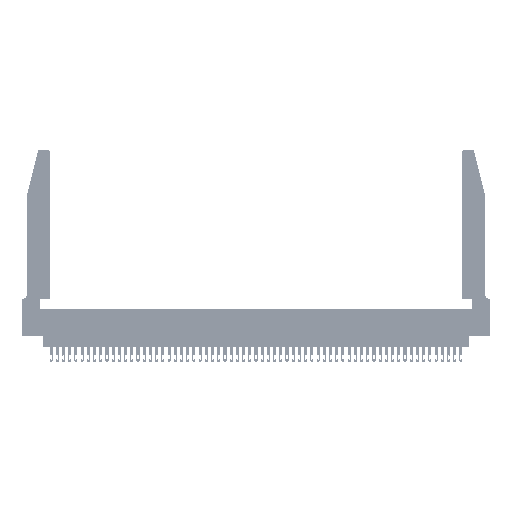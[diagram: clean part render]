
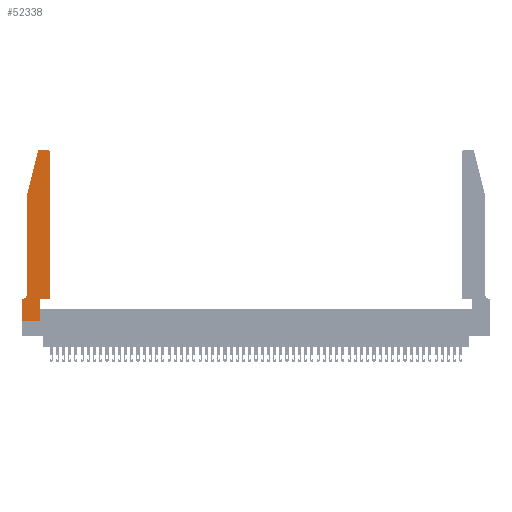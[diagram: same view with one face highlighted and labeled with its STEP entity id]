
A CAD part, top view. The second image highlights one B-rep face of the part: STEP entity #52338.
In plain terms, the highlighted planar face has unit normal (0, 0, 1).
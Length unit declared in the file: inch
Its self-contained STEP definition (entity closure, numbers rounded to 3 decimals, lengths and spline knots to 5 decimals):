
#131 = VECTOR ( 'NONE', #1673, 39.37008 ) ;
#304 = CIRCLE ( 'NONE', #23443, 0.03 ) ;
#316 = ORIENTED_EDGE ( 'NONE', *, *, #53068, .T. ) ;
#607 = CARTESIAN_POINT ( 'NONE',  ( 0.4505, 0.35, 0.37 ) ) ;
#692 = VERTEX_POINT ( 'NONE', #607 ) ;
#1116 = LINE ( 'NONE', #1582, #50040 ) ;
#1502 = DIRECTION ( 'NONE',  ( 1., 0., 0. ) ) ;
#1566 = EDGE_CURVE ( 'NONE', #12798, #52651, #2098, .T. ) ;
#1578 = EDGE_CURVE ( 'NONE', #48732, #12798, #47738, .T. ) ;
#1582 = CARTESIAN_POINT ( 'NONE',  ( 0., 0., 0.37 ) ) ;
#1673 = DIRECTION ( 'NONE',  ( -0.239, -0.971, 0. ) ) ;
#2098 = CIRCLE ( 'NONE', #34013, 0.03 ) ;
#4130 = EDGE_CURVE ( 'NONE', #20633, #27857, #36004, .T. ) ;
#5113 = CARTESIAN_POINT ( 'NONE',  ( 0.2865, 0.35, 0.37 ) ) ;
#8477 = ORIENTED_EDGE ( 'NONE', *, *, #46978, .T. ) ;
#8894 = VERTEX_POINT ( 'NONE', #49794 ) ;
#9693 = LINE ( 'NONE', #29654, #25375 ) ;
#10575 = CARTESIAN_POINT ( 'NONE',  ( 0.2865, 0., 0.37 ) ) ;
#11059 = CARTESIAN_POINT ( 'NONE',  ( 0., 0.35, 0.37 ) ) ;
#11679 = CARTESIAN_POINT ( 'NONE',  ( 0.2865, 0.35, 0.37 ) ) ;
#12298 = EDGE_CURVE ( 'NONE', #30805, #37661, #46729, .T. ) ;
#12798 = VERTEX_POINT ( 'NONE', #39638 ) ;
#13905 = FACE_OUTER_BOUND ( 'NONE', #34960, .T. ) ;
#14995 = VERTEX_POINT ( 'NONE', #46528 ) ;
#16241 = CARTESIAN_POINT ( 'NONE',  ( 0., 0.35, 0.37 ) ) ;
#16533 = CARTESIAN_POINT ( 'NONE',  ( 0.4505, 0.35, 0.37 ) ) ;
#17846 = VECTOR ( 'NONE', #1502, 39.37008 ) ;
#19069 = DIRECTION ( 'NONE',  ( 0., -1., 0. ) ) ;
#19104 = ORIENTED_EDGE ( 'NONE', *, *, #1566, .T. ) ;
#19164 = CARTESIAN_POINT ( 'NONE',  ( 0.0055, 0.42, 0.37 ) ) ;
#19542 = ORIENTED_EDGE ( 'NONE', *, *, #33778, .T. ) ;
#19717 = DIRECTION ( 'NONE',  ( -1., 0., 0. ) ) ;
#20386 = VECTOR ( 'NONE', #51814, 39.37008 ) ;
#20387 = ORIENTED_EDGE ( 'NONE', *, *, #21474, .T. ) ;
#20444 = DIRECTION ( 'NONE',  ( 1., 0., 0. ) ) ;
#20633 = VERTEX_POINT ( 'NONE', #53110 ) ;
#20635 = DIRECTION ( 'NONE',  ( 1., 0., 0. ) ) ;
#20976 = DIRECTION ( 'NONE',  ( 0., 0., 1. ) ) ;
#21041 = LINE ( 'NONE', #43050, #131 ) ;
#21474 = EDGE_CURVE ( 'NONE', #52651, #30805, #21041, .T. ) ;
#23443 = AXIS2_PLACEMENT_3D ( 'NONE', #49747, #50461, #50110 ) ;
#23986 = ORIENTED_EDGE ( 'NONE', *, *, #4130, .T. ) ;
#24765 = DIRECTION ( 'NONE',  ( 1., 0., 0. ) ) ;
#25063 = EDGE_CURVE ( 'NONE', #8894, #42258, #48500, .T. ) ;
#25287 = DIRECTION ( 'NONE',  ( 0., 1., 0. ) ) ;
#25375 = VECTOR ( 'NONE', #25287, 39.37008 ) ;
#25563 = VECTOR ( 'NONE', #19717, 39.37008 ) ;
#25786 = ORIENTED_EDGE ( 'NONE', *, *, #25063, .T. ) ;
#26213 = LINE ( 'NONE', #16533, #35977 ) ;
#26375 = ORIENTED_EDGE ( 'NONE', *, *, #12298, .T. ) ;
#27857 = VERTEX_POINT ( 'NONE', #11059 ) ;
#28106 = EDGE_CURVE ( 'NONE', #692, #14995, #9693, .T. ) ;
#29121 = VERTEX_POINT ( 'NONE', #11679 ) ;
#29248 = ORIENTED_EDGE ( 'NONE', *, *, #41153, .T. ) ;
#29654 = CARTESIAN_POINT ( 'NONE',  ( 0.4505, 0.35, 0.37 ) ) ;
#30805 = VERTEX_POINT ( 'NONE', #31162 ) ;
#31162 = CARTESIAN_POINT ( 'NONE',  ( 0.0755, 2., 0.37 ) ) ;
#32603 = CIRCLE ( 'NONE', #42504, 0.07 ) ;
#33019 = CARTESIAN_POINT ( 'NONE',  ( 0.284, 2.72, 0.37 ) ) ;
#33319 = ORIENTED_EDGE ( 'NONE', *, *, #1578, .T. ) ;
#33668 = ORIENTED_EDGE ( 'NONE', *, *, #43805, .T. ) ;
#33778 = EDGE_CURVE ( 'NONE', #42258, #29121, #51912, .T. ) ;
#34013 = AXIS2_PLACEMENT_3D ( 'NONE', #33019, #41384, #20635 ) ;
#34960 = EDGE_LOOP ( 'NONE', ( #33319, #19104, #20387, #26375, #33668, #23986, #29248, #25786, #19542, #316, #50318, #8477 ) ) ;
#35565 = CARTESIAN_POINT ( 'NONE',  ( 0.0755, 0.35, 0.37 ) ) ;
#35977 = VECTOR ( 'NONE', #24765, 39.37008 ) ;
#36004 = LINE ( 'NONE', #35565, #20386 ) ;
#37661 = VERTEX_POINT ( 'NONE', #50628 ) ;
#38705 = CARTESIAN_POINT ( 'NONE',  ( 0., 0., 0.37 ) ) ;
#39638 = CARTESIAN_POINT ( 'NONE',  ( 0.284, 2.75, 0.37 ) ) ;
#40929 = DIRECTION ( 'NONE',  ( 0., -1., 0. ) ) ;
#41153 = EDGE_CURVE ( 'NONE', #27857, #8894, #1116, .T. ) ;
#41384 = DIRECTION ( 'NONE',  ( 0., 0., 1. ) ) ;
#42258 = VERTEX_POINT ( 'NONE', #10575 ) ;
#42504 = AXIS2_PLACEMENT_3D ( 'NONE', #19164, #48508, #48345 ) ;
#42813 = CARTESIAN_POINT ( 'NONE',  ( 0.25487, 2.72718, 0.37 ) ) ;
#43050 = CARTESIAN_POINT ( 'NONE',  ( 0.0755, 2., 0.37 ) ) ;
#43805 = EDGE_CURVE ( 'NONE', #37661, #20633, #32603, .T. ) ;
#44979 = CARTESIAN_POINT ( 'NONE',  ( 0.0755, 2., 0.37 ) ) ;
#45943 = PLANE ( 'NONE',  #53332 ) ;
#46528 = CARTESIAN_POINT ( 'NONE',  ( 0.4505, 2.72, 0.37 ) ) ;
#46729 = LINE ( 'NONE', #44979, #51285 ) ;
#46978 = EDGE_CURVE ( 'NONE', #14995, #48732, #304, .T. ) ;
#47738 = LINE ( 'NONE', #52754, #25563 ) ;
#48345 = DIRECTION ( 'NONE',  ( -1., 0., 0. ) ) ;
#48500 = LINE ( 'NONE', #38705, #17846 ) ;
#48508 = DIRECTION ( 'NONE',  ( 0., 0., -1. ) ) ;
#48732 = VERTEX_POINT ( 'NONE', #50054 ) ;
#49483 = DIRECTION ( 'NONE',  ( 0., 1., 0. ) ) ;
#49747 = CARTESIAN_POINT ( 'NONE',  ( 0.4205, 2.72, 0.37 ) ) ;
#49794 = CARTESIAN_POINT ( 'NONE',  ( 0., 0., 0.37 ) ) ;
#49942 = VECTOR ( 'NONE', #49483, 39.37008 ) ;
#50040 = VECTOR ( 'NONE', #19069, 39.37008 ) ;
#50054 = CARTESIAN_POINT ( 'NONE',  ( 0.4205, 2.75, 0.37 ) ) ;
#50110 = DIRECTION ( 'NONE',  ( 1., 0., 0. ) ) ;
#50318 = ORIENTED_EDGE ( 'NONE', *, *, #28106, .T. ) ;
#50461 = DIRECTION ( 'NONE',  ( 0., 0., 1. ) ) ;
#50628 = CARTESIAN_POINT ( 'NONE',  ( 0.0755, 0.42, 0.37 ) ) ;
#51285 = VECTOR ( 'NONE', #40929, 39.37008 ) ;
#51814 = DIRECTION ( 'NONE',  ( -1., 0., 0. ) ) ;
#51912 = LINE ( 'NONE', #5113, #49942 ) ;
#52338 = ADVANCED_FACE ( 'NONE', ( #13905 ), #45943, .T. ) ;
#52651 = VERTEX_POINT ( 'NONE', #42813 ) ;
#52754 = CARTESIAN_POINT ( 'NONE',  ( 0.2605, 2.75, 0.37 ) ) ;
#53068 = EDGE_CURVE ( 'NONE', #29121, #692, #26213, .T. ) ;
#53110 = CARTESIAN_POINT ( 'NONE',  ( 0.0055, 0.35, 0.37 ) ) ;
#53332 = AXIS2_PLACEMENT_3D ( 'NONE', #16241, #20976, #20444 ) ;
